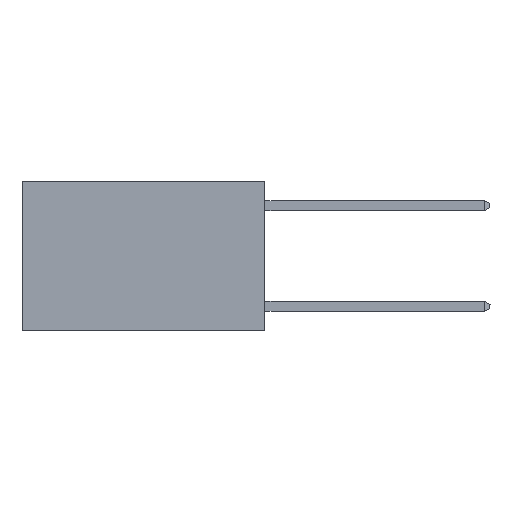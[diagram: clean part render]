
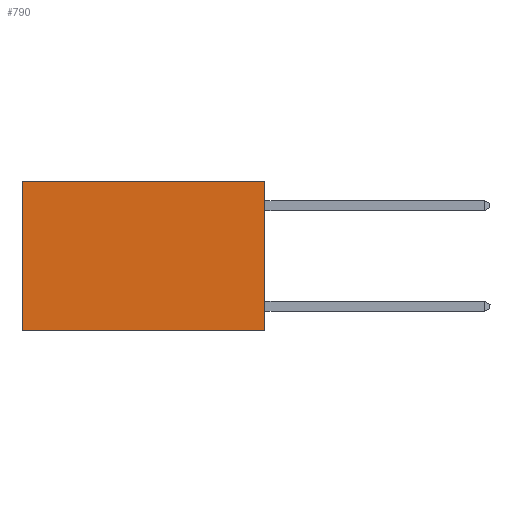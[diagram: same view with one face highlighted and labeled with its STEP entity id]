
A CAD part, left-side view. The second image highlights one B-rep face of the part: STEP entity #790.
In plain terms, the highlighted planar face has unit normal (-1, 0, 0).
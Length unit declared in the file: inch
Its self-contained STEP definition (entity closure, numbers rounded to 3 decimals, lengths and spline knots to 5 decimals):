
#627 = VECTOR ( 'NONE', #9349, 39.37008 ) ;
#790 = ADVANCED_FACE ( 'NONE', ( #3143 ), #17538, .F. ) ;
#2002 = VERTEX_POINT ( 'NONE', #10087 ) ;
#2862 = CARTESIAN_POINT ( 'NONE',  ( 0.2625, 0., 0. ) ) ;
#3143 = FACE_OUTER_BOUND ( 'NONE', #6330, .T. ) ;
#3808 = ORIENTED_EDGE ( 'NONE', *, *, #8566, .F. ) ;
#3895 = DIRECTION ( 'NONE',  ( 0., 0., -1. ) ) ;
#5339 = VERTEX_POINT ( 'NONE', #6225 ) ;
#5434 = CARTESIAN_POINT ( 'NONE',  ( 0.2625, 0., -0.37 ) ) ;
#6165 = ORIENTED_EDGE ( 'NONE', *, *, #15456, .T. ) ;
#6225 = CARTESIAN_POINT ( 'NONE',  ( 0.2625, 0.6, 0. ) ) ;
#6330 = EDGE_LOOP ( 'NONE', ( #21044, #3808, #25027, #6165 ) ) ;
#7047 = DIRECTION ( 'NONE',  ( 1., 0., 0. ) ) ;
#7168 = CARTESIAN_POINT ( 'NONE',  ( 0.2625, 0.6, 0. ) ) ;
#7222 = VERTEX_POINT ( 'NONE', #15358 ) ;
#8566 = EDGE_CURVE ( 'NONE', #16463, #7222, #11048, .T. ) ;
#9349 = DIRECTION ( 'NONE',  ( 0., 1., 0. ) ) ;
#10087 = CARTESIAN_POINT ( 'NONE',  ( 0.2625, 0., 0. ) ) ;
#10434 = CARTESIAN_POINT ( 'NONE',  ( 0.2625, 0., 0. ) ) ;
#11048 = LINE ( 'NONE', #5434, #627 ) ;
#12192 = VECTOR ( 'NONE', #3895, 39.37008 ) ;
#12943 = DIRECTION ( 'NONE',  ( 0., 0., -1. ) ) ;
#13081 = DIRECTION ( 'NONE',  ( 0., 0., -1. ) ) ;
#14215 = EDGE_CURVE ( 'NONE', #5339, #7222, #17374, .T. ) ;
#15124 = EDGE_CURVE ( 'NONE', #2002, #16463, #16724, .T. ) ;
#15183 = LINE ( 'NONE', #2862, #20288 ) ;
#15358 = CARTESIAN_POINT ( 'NONE',  ( 0.2625, 0.6, -0.37 ) ) ;
#15456 = EDGE_CURVE ( 'NONE', #2002, #5339, #15183, .T. ) ;
#15565 = CARTESIAN_POINT ( 'NONE',  ( 0.2625, 0., 0. ) ) ;
#16463 = VERTEX_POINT ( 'NONE', #17809 ) ;
#16724 = LINE ( 'NONE', #15565, #12192 ) ;
#16775 = VECTOR ( 'NONE', #13081, 39.37008 ) ;
#17374 = LINE ( 'NONE', #7168, #16775 ) ;
#17538 = PLANE ( 'NONE',  #22522 ) ;
#17809 = CARTESIAN_POINT ( 'NONE',  ( 0.2625, 0., -0.37 ) ) ;
#18419 = DIRECTION ( 'NONE',  ( 0., 1., 0. ) ) ;
#20288 = VECTOR ( 'NONE', #18419, 39.37008 ) ;
#21044 = ORIENTED_EDGE ( 'NONE', *, *, #14215, .T. ) ;
#22522 = AXIS2_PLACEMENT_3D ( 'NONE', #10434, #7047, #12943 ) ;
#25027 = ORIENTED_EDGE ( 'NONE', *, *, #15124, .F. ) ;
